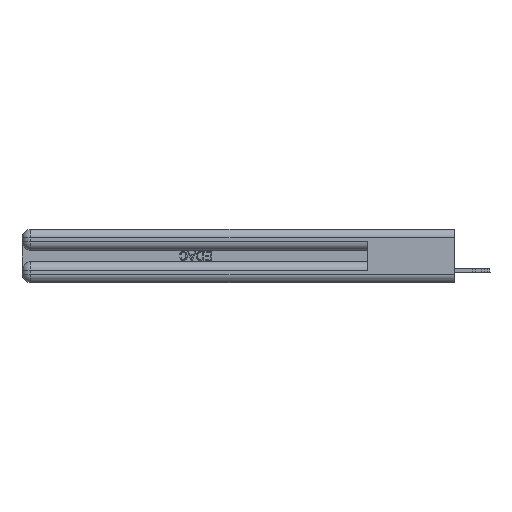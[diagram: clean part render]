
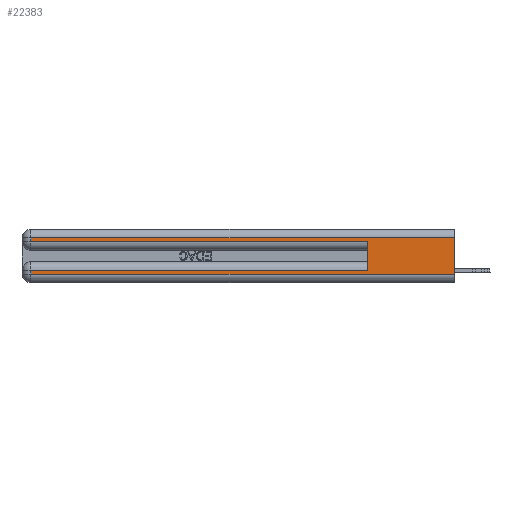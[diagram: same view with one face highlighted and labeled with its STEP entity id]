
A CAD part, left-side view. The second image highlights one B-rep face of the part: STEP entity #22383.
In plain terms, the highlighted planar face has unit normal (-1, 0, 0).
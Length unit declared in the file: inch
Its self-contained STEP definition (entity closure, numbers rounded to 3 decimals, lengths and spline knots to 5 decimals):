
#246 = ORIENTED_EDGE ( 'NONE', *, *, #30290, .F. ) ;
#1366 = ORIENTED_EDGE ( 'NONE', *, *, #19322, .T. ) ;
#1456 = CARTESIAN_POINT ( 'NONE',  ( 0., 0., 0.285 ) ) ;
#1877 = LINE ( 'NONE', #1456, #11850 ) ;
#2008 = DIRECTION ( 'NONE',  ( 0., -1., 0. ) ) ;
#2100 = VERTEX_POINT ( 'NONE', #24073 ) ;
#2601 = VECTOR ( 'NONE', #12251, 39.37008 ) ;
#3649 = DIRECTION ( 'NONE',  ( 1., 0., 0. ) ) ;
#4361 = LINE ( 'NONE', #8267, #29255 ) ;
#5809 = CARTESIAN_POINT ( 'NONE',  ( 0., 2.94, 0.06 ) ) ;
#6408 = VERTEX_POINT ( 'NONE', #11861 ) ;
#6900 = DIRECTION ( 'NONE',  ( 0., 0., 1. ) ) ;
#7267 = FACE_OUTER_BOUND ( 'NONE', #29247, .T. ) ;
#7997 = VERTEX_POINT ( 'NONE', #33878 ) ;
#8267 = CARTESIAN_POINT ( 'NONE',  ( 0., 0., 0.31 ) ) ;
#8354 = DIRECTION ( 'NONE',  ( 0., 0., -1. ) ) ;
#8365 = LINE ( 'NONE', #26060, #10307 ) ;
#8469 = EDGE_CURVE ( 'NONE', #7997, #36630, #1877, .T. ) ;
#8502 = EDGE_CURVE ( 'NONE', #32518, #6408, #4361, .T. ) ;
#9844 = VECTOR ( 'NONE', #17549, 39.37008 ) ;
#10307 = VECTOR ( 'NONE', #32697, 39.37008 ) ;
#11850 = VECTOR ( 'NONE', #2008, 39.37008 ) ;
#11861 = CARTESIAN_POINT ( 'NONE',  ( 0., 2.94, 0.31 ) ) ;
#12251 = DIRECTION ( 'NONE',  ( 0., 0., -1. ) ) ;
#13132 = VERTEX_POINT ( 'NONE', #5809 ) ;
#13300 = DIRECTION ( 'NONE',  ( 0., 0., -1. ) ) ;
#17426 = CARTESIAN_POINT ( 'NONE',  ( 0., 2.94, 0.37 ) ) ;
#17549 = DIRECTION ( 'NONE',  ( 0., 1., 0. ) ) ;
#19322 = EDGE_CURVE ( 'NONE', #6408, #7997, #28007, .T. ) ;
#19795 = CARTESIAN_POINT ( 'NONE',  ( 0., 0., 0.37 ) ) ;
#19951 = VECTOR ( 'NONE', #6900, 39.37008 ) ;
#20293 = LINE ( 'NONE', #33130, #9844 ) ;
#20592 = CARTESIAN_POINT ( 'NONE',  ( 0., 0.6, 0.285 ) ) ;
#20865 = ORIENTED_EDGE ( 'NONE', *, *, #8502, .T. ) ;
#20972 = CARTESIAN_POINT ( 'NONE',  ( 0., 2.94, 0.37 ) ) ;
#21033 = DIRECTION ( 'NONE',  ( 0., 1., 0. ) ) ;
#21265 = EDGE_CURVE ( 'NONE', #32334, #35000, #20293, .T. ) ;
#21448 = EDGE_CURVE ( 'NONE', #35000, #13132, #38086, .T. ) ;
#21609 = CARTESIAN_POINT ( 'NONE',  ( 0., 0., 0.31 ) ) ;
#21755 = AXIS2_PLACEMENT_3D ( 'NONE', #19795, #3649, #22998 ) ;
#22383 = ADVANCED_FACE ( 'NONE', ( #7267 ), #35326, .F. ) ;
#22512 = CARTESIAN_POINT ( 'NONE',  ( 0., 0., 0.37 ) ) ;
#22998 = DIRECTION ( 'NONE',  ( 0., 0., -1. ) ) ;
#23426 = LINE ( 'NONE', #35195, #19951 ) ;
#23664 = ORIENTED_EDGE ( 'NONE', *, *, #8469, .T. ) ;
#24073 = CARTESIAN_POINT ( 'NONE',  ( 0., 0., 0.06 ) ) ;
#24971 = EDGE_CURVE ( 'NONE', #32518, #2100, #30494, .T. ) ;
#26060 = CARTESIAN_POINT ( 'NONE',  ( 0., 0., 0.06 ) ) ;
#26505 = CARTESIAN_POINT ( 'NONE',  ( 0., 0.6, 0.085 ) ) ;
#28007 = LINE ( 'NONE', #17426, #2601 ) ;
#29247 = EDGE_LOOP ( 'NONE', ( #38520, #20865, #1366, #23664, #246, #37639, #37304, #35461 ) ) ;
#29255 = VECTOR ( 'NONE', #21033, 39.37008 ) ;
#30290 = EDGE_CURVE ( 'NONE', #32334, #36630, #23426, .T. ) ;
#30494 = LINE ( 'NONE', #22512, #33471 ) ;
#32334 = VERTEX_POINT ( 'NONE', #26505 ) ;
#32518 = VERTEX_POINT ( 'NONE', #21609 ) ;
#32697 = DIRECTION ( 'NONE',  ( 0., -1., 0. ) ) ;
#32800 = EDGE_CURVE ( 'NONE', #13132, #2100, #8365, .T. ) ;
#33130 = CARTESIAN_POINT ( 'NONE',  ( 0., 0., 0.085 ) ) ;
#33471 = VECTOR ( 'NONE', #13300, 39.37008 ) ;
#33878 = CARTESIAN_POINT ( 'NONE',  ( 0., 2.94, 0.285 ) ) ;
#35000 = VERTEX_POINT ( 'NONE', #35174 ) ;
#35174 = CARTESIAN_POINT ( 'NONE',  ( 0., 2.94, 0.085 ) ) ;
#35195 = CARTESIAN_POINT ( 'NONE',  ( 0., 0.6, 0.145 ) ) ;
#35326 = PLANE ( 'NONE',  #21755 ) ;
#35461 = ORIENTED_EDGE ( 'NONE', *, *, #32800, .T. ) ;
#36109 = VECTOR ( 'NONE', #8354, 39.37008 ) ;
#36630 = VERTEX_POINT ( 'NONE', #20592 ) ;
#37304 = ORIENTED_EDGE ( 'NONE', *, *, #21448, .T. ) ;
#37639 = ORIENTED_EDGE ( 'NONE', *, *, #21265, .T. ) ;
#38086 = LINE ( 'NONE', #20972, #36109 ) ;
#38520 = ORIENTED_EDGE ( 'NONE', *, *, #24971, .F. ) ;
